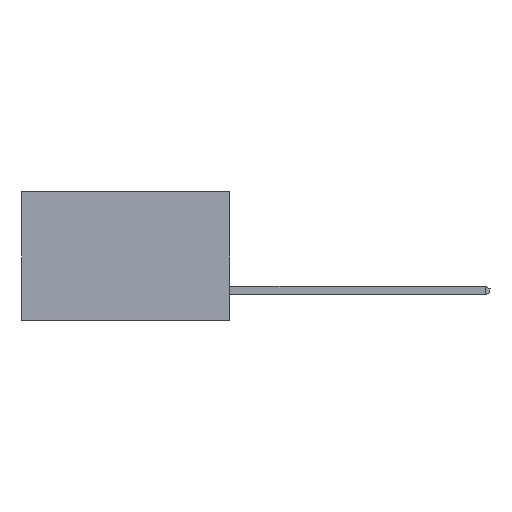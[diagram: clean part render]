
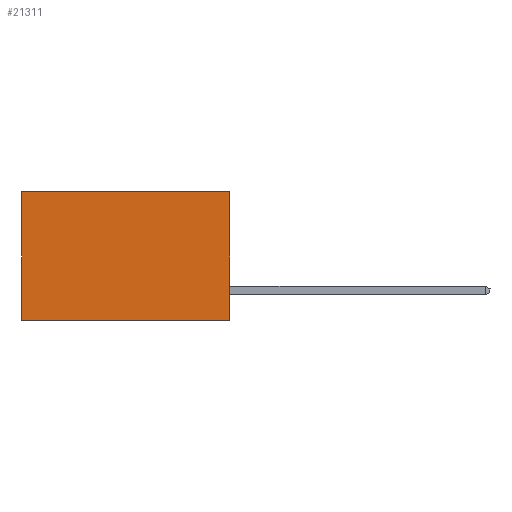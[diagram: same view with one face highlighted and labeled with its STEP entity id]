
A CAD part, left-side view. The second image highlights one B-rep face of the part: STEP entity #21311.
In plain terms, the highlighted planar face has unit normal (-1, 0, 0).
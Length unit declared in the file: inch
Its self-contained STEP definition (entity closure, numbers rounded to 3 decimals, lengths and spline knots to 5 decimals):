
#576 = LINE ( 'NONE', #23863, #23568 ) ;
#993 = PLANE ( 'NONE',  #15139 ) ;
#1350 = CARTESIAN_POINT ( 'NONE',  ( 0.2615, 0., -0.37 ) ) ;
#1432 = VECTOR ( 'NONE', #21760, 39.37008 ) ;
#1511 = VECTOR ( 'NONE', #2011, 39.37008 ) ;
#2011 = DIRECTION ( 'NONE',  ( 0., 1., 0. ) ) ;
#2505 = DIRECTION ( 'NONE',  ( 0., 0., -1. ) ) ;
#3217 = CARTESIAN_POINT ( 'NONE',  ( 0.2615, 0.6, -0.37 ) ) ;
#3858 = ORIENTED_EDGE ( 'NONE', *, *, #18596, .T. ) ;
#5151 = ORIENTED_EDGE ( 'NONE', *, *, #10186, .F. ) ;
#5500 = DIRECTION ( 'NONE',  ( 0., 0., -1. ) ) ;
#6435 = CARTESIAN_POINT ( 'NONE',  ( 0.2615, 0.6, 0. ) ) ;
#6492 = ORIENTED_EDGE ( 'NONE', *, *, #22038, .T. ) ;
#7728 = ORIENTED_EDGE ( 'NONE', *, *, #8264, .F. ) ;
#8046 = LINE ( 'NONE', #19657, #16803 ) ;
#8264 = EDGE_CURVE ( 'NONE', #9532, #23833, #11545, .T. ) ;
#9407 = EDGE_LOOP ( 'NONE', ( #3858, #7728, #5151, #6492 ) ) ;
#9532 = VERTEX_POINT ( 'NONE', #1350 ) ;
#10186 = EDGE_CURVE ( 'NONE', #14883, #9532, #8046, .T. ) ;
#10557 = FACE_OUTER_BOUND ( 'NONE', #9407, .T. ) ;
#11290 = DIRECTION ( 'NONE',  ( 1., 0., 0. ) ) ;
#11545 = LINE ( 'NONE', #15157, #1511 ) ;
#14883 = VERTEX_POINT ( 'NONE', #24714 ) ;
#15139 = AXIS2_PLACEMENT_3D ( 'NONE', #16649, #11290, #5500 ) ;
#15157 = CARTESIAN_POINT ( 'NONE',  ( 0.2615, 0., -0.37 ) ) ;
#16504 = CARTESIAN_POINT ( 'NONE',  ( 0.2615, 0.6, -0.37 ) ) ;
#16649 = CARTESIAN_POINT ( 'NONE',  ( 0.2615, 0., -0.37 ) ) ;
#16803 = VECTOR ( 'NONE', #2505, 39.37008 ) ;
#18596 = EDGE_CURVE ( 'NONE', #21211, #23833, #19877, .T. ) ;
#19657 = CARTESIAN_POINT ( 'NONE',  ( 0.2615, 0., -0.37 ) ) ;
#19877 = LINE ( 'NONE', #3217, #1432 ) ;
#21211 = VERTEX_POINT ( 'NONE', #6435 ) ;
#21311 = ADVANCED_FACE ( 'NONE', ( #10557 ), #993, .F. ) ;
#21760 = DIRECTION ( 'NONE',  ( 0., 0., -1. ) ) ;
#22038 = EDGE_CURVE ( 'NONE', #14883, #21211, #576, .T. ) ;
#23568 = VECTOR ( 'NONE', #23629, 39.37008 ) ;
#23629 = DIRECTION ( 'NONE',  ( 0., 1., 0. ) ) ;
#23833 = VERTEX_POINT ( 'NONE', #16504 ) ;
#23863 = CARTESIAN_POINT ( 'NONE',  ( 0.2615, 0., 0. ) ) ;
#24714 = CARTESIAN_POINT ( 'NONE',  ( 0.2615, 0., 0. ) ) ;
